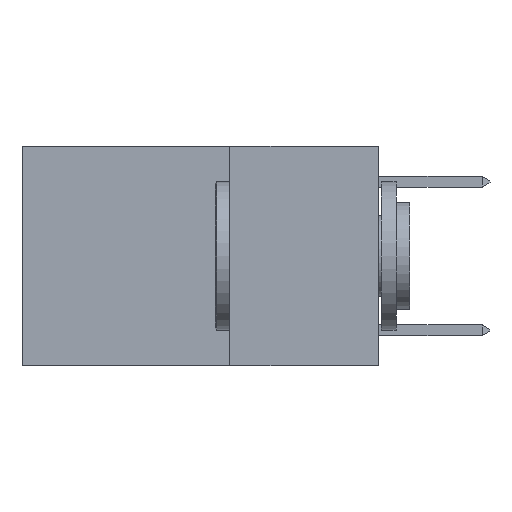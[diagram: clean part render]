
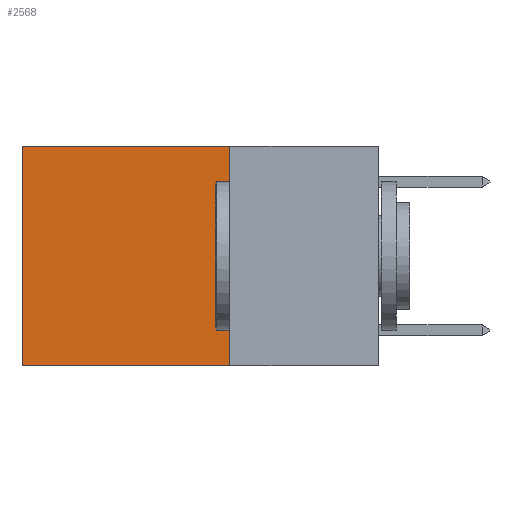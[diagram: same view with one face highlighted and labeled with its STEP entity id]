
A CAD part, left-side view. The second image highlights one B-rep face of the part: STEP entity #2568.
In plain terms, the highlighted planar face has unit normal (-1, 0, 0).
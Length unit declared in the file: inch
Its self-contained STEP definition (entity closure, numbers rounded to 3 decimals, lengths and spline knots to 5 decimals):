
#479 = CARTESIAN_POINT ( 'NONE',  ( 0.2625, 0.25, -0.37 ) ) ;
#585 = EDGE_CURVE ( 'NONE', #1131, #6304, #3668, .T. ) ;
#1131 = VERTEX_POINT ( 'NONE', #3803 ) ;
#1175 = CARTESIAN_POINT ( 'NONE',  ( 0.2625, 0.6, 0. ) ) ;
#1551 = CARTESIAN_POINT ( 'NONE',  ( 0.2625, 0.25, -0.37 ) ) ;
#1578 = EDGE_CURVE ( 'NONE', #6304, #5524, #4809, .T. ) ;
#1650 = ORIENTED_EDGE ( 'NONE', *, *, #5069, .F. ) ;
#2036 = FACE_OUTER_BOUND ( 'NONE', #2245, .T. ) ;
#2245 = EDGE_LOOP ( 'NONE', ( #6557, #1650, #4951, #5506 ) ) ;
#2308 = VECTOR ( 'NONE', #4347, 39.37008 ) ;
#2568 = ADVANCED_FACE ( 'NONE', ( #2036 ), #6999, .F. ) ;
#2895 = CARTESIAN_POINT ( 'NONE',  ( 0.2625, 0.25, 0. ) ) ;
#3417 = VECTOR ( 'NONE', #9310, 39.37008 ) ;
#3434 = LINE ( 'NONE', #7768, #7673 ) ;
#3668 = LINE ( 'NONE', #2895, #2308 ) ;
#3803 = CARTESIAN_POINT ( 'NONE',  ( 0.2625, 0.25, 0. ) ) ;
#3915 = VECTOR ( 'NONE', #7642, 39.37008 ) ;
#4347 = DIRECTION ( 'NONE',  ( 0., 1., 0. ) ) ;
#4809 = LINE ( 'NONE', #1175, #3915 ) ;
#4951 = ORIENTED_EDGE ( 'NONE', *, *, #7920, .F. ) ;
#5059 = CARTESIAN_POINT ( 'NONE',  ( 0.2625, 0.6, 0. ) ) ;
#5069 = EDGE_CURVE ( 'NONE', #8148, #5524, #6537, .T. ) ;
#5506 = ORIENTED_EDGE ( 'NONE', *, *, #585, .T. ) ;
#5524 = VERTEX_POINT ( 'NONE', #8974 ) ;
#5652 = CARTESIAN_POINT ( 'NONE',  ( 0.2625, 0.25, 0. ) ) ;
#6304 = VERTEX_POINT ( 'NONE', #5059 ) ;
#6322 = DIRECTION ( 'NONE',  ( 1., 0., 0. ) ) ;
#6537 = LINE ( 'NONE', #479, #3417 ) ;
#6557 = ORIENTED_EDGE ( 'NONE', *, *, #1578, .T. ) ;
#6999 = PLANE ( 'NONE',  #8419 ) ;
#7642 = DIRECTION ( 'NONE',  ( 0., 0., -1. ) ) ;
#7673 = VECTOR ( 'NONE', #8642, 39.37008 ) ;
#7768 = CARTESIAN_POINT ( 'NONE',  ( 0.2625, 0.25, 0. ) ) ;
#7920 = EDGE_CURVE ( 'NONE', #1131, #8148, #3434, .T. ) ;
#8148 = VERTEX_POINT ( 'NONE', #1551 ) ;
#8419 = AXIS2_PLACEMENT_3D ( 'NONE', #5652, #6322, #9336 ) ;
#8642 = DIRECTION ( 'NONE',  ( 0., 0., -1. ) ) ;
#8974 = CARTESIAN_POINT ( 'NONE',  ( 0.2625, 0.6, -0.37 ) ) ;
#9310 = DIRECTION ( 'NONE',  ( 0., 1., 0. ) ) ;
#9336 = DIRECTION ( 'NONE',  ( 0., 0., -1. ) ) ;
